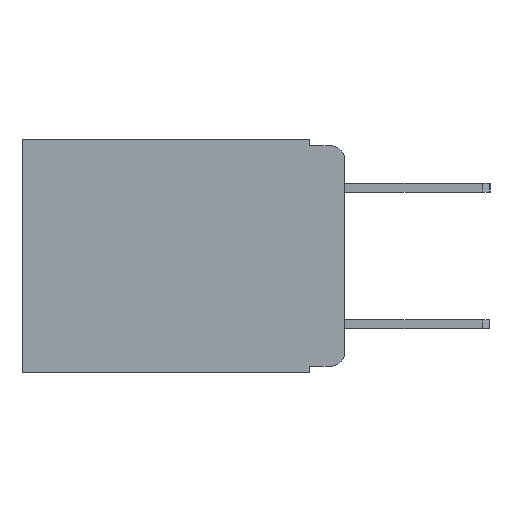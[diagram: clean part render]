
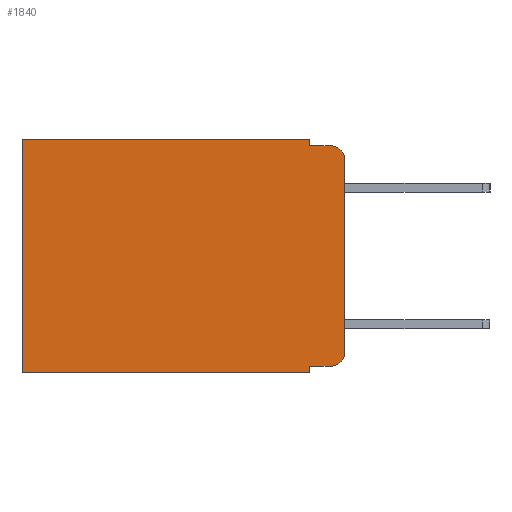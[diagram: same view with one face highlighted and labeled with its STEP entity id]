
A CAD part, left-side view. The second image highlights one B-rep face of the part: STEP entity #1840.
In plain terms, the highlighted planar face has unit normal (-1, 0, 0).
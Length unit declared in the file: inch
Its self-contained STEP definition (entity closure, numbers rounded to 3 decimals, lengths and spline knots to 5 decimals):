
#321 = ORIENTED_EDGE ( 'NONE', *, *, #17879, .T. ) ;
#538 = ORIENTED_EDGE ( 'NONE', *, *, #2535, .T. ) ;
#560 = EDGE_CURVE ( 'NONE', #4460, #9478, #13336, .T. ) ;
#1065 = DIRECTION ( 'NONE',  ( -1., 0., 0. ) ) ;
#1260 = CARTESIAN_POINT ( 'NONE',  ( 0.298, 0.051, 0. ) ) ;
#1289 = ORIENTED_EDGE ( 'NONE', *, *, #3082, .F. ) ;
#1508 = ORIENTED_EDGE ( 'NONE', *, *, #16842, .F. ) ;
#1840 = ADVANCED_FACE ( 'NONE', ( #6047 ), #12514, .F. ) ;
#1930 = ORIENTED_EDGE ( 'NONE', *, *, #10732, .T. ) ;
#2207 = DIRECTION ( 'NONE',  ( 0., 0., -1. ) ) ;
#2435 = AXIS2_PLACEMENT_3D ( 'NONE', #12482, #1065, #2207 ) ;
#2487 = VERTEX_POINT ( 'NONE', #9283 ) ;
#2535 = EDGE_CURVE ( 'NONE', #7616, #2487, #5791, .T. ) ;
#2901 = CARTESIAN_POINT ( 'NONE',  ( 0.298, 0.02, -0.333 ) ) ;
#2930 = ORIENTED_EDGE ( 'NONE', *, *, #5028, .T. ) ;
#2980 = DIRECTION ( 'NONE',  ( 0., 0., -1. ) ) ;
#3056 = EDGE_CURVE ( 'NONE', #16772, #5323, #15307, .T. ) ;
#3082 = EDGE_CURVE ( 'NONE', #16664, #2487, #7813, .T. ) ;
#3598 = CARTESIAN_POINT ( 'NONE',  ( 0.298, 0.051, -0.01 ) ) ;
#3808 = VECTOR ( 'NONE', #9976, 39.37008 ) ;
#4330 = LINE ( 'NONE', #16898, #7818 ) ;
#4460 = VERTEX_POINT ( 'NONE', #10385 ) ;
#4520 = CARTESIAN_POINT ( 'NONE',  ( 0.298, 0.051, 0. ) ) ;
#5028 = EDGE_CURVE ( 'NONE', #5469, #15815, #16810, .T. ) ;
#5250 = EDGE_LOOP ( 'NONE', ( #15176, #15580, #11083, #11491, #321, #538, #1289, #1508, #1930, #2930 ) ) ;
#5323 = VERTEX_POINT ( 'NONE', #12363 ) ;
#5452 = EDGE_CURVE ( 'NONE', #4460, #15815, #17604, .T. ) ;
#5469 = VERTEX_POINT ( 'NONE', #2901 ) ;
#5500 = VECTOR ( 'NONE', #2980, 39.37008 ) ;
#5740 = CARTESIAN_POINT ( 'NONE',  ( 0.298, 0.051, -0.343 ) ) ;
#5791 = LINE ( 'NONE', #6380, #9594 ) ;
#6042 = CARTESIAN_POINT ( 'NONE',  ( 0.298, 0., 0. ) ) ;
#6047 = FACE_OUTER_BOUND ( 'NONE', #5250, .T. ) ;
#6196 = EDGE_CURVE ( 'NONE', #5323, #9478, #10056, .T. ) ;
#6380 = CARTESIAN_POINT ( 'NONE',  ( 0.298, 0.473, 0. ) ) ;
#6411 = DIRECTION ( 'NONE',  ( 0., 0., -1. ) ) ;
#6640 = CARTESIAN_POINT ( 'NONE',  ( 0.298, 0., -0.313 ) ) ;
#6950 = CARTESIAN_POINT ( 'NONE',  ( 0.298, 0.051, 0. ) ) ;
#7023 = VECTOR ( 'NONE', #14177, 39.37008 ) ;
#7038 = DIRECTION ( 'NONE',  ( 0., 0., -1. ) ) ;
#7078 = VECTOR ( 'NONE', #9810, 39.37008 ) ;
#7616 = VERTEX_POINT ( 'NONE', #15368 ) ;
#7813 = LINE ( 'NONE', #14755, #3808 ) ;
#7818 = VECTOR ( 'NONE', #9133, 39.37008 ) ;
#8032 = AXIS2_PLACEMENT_3D ( 'NONE', #16397, #12651, #12625 ) ;
#8724 = VECTOR ( 'NONE', #7038, 39.37008 ) ;
#9133 = DIRECTION ( 'NONE',  ( 0., -1., 0. ) ) ;
#9283 = CARTESIAN_POINT ( 'NONE',  ( 0.298, 0.473, -0.343 ) ) ;
#9478 = VERTEX_POINT ( 'NONE', #14323 ) ;
#9594 = VECTOR ( 'NONE', #6411, 39.37008 ) ;
#9645 = VECTOR ( 'NONE', #12471, 39.37008 ) ;
#9765 = LINE ( 'NONE', #4520, #5500 ) ;
#9810 = DIRECTION ( 'NONE',  ( 0., 1., 0. ) ) ;
#9976 = DIRECTION ( 'NONE',  ( 0., 1., 0. ) ) ;
#10056 = LINE ( 'NONE', #3598, #9645 ) ;
#10376 = DIRECTION ( 'NONE',  ( -1., 0., 0. ) ) ;
#10385 = CARTESIAN_POINT ( 'NONE',  ( 0.298, 0., -0.03 ) ) ;
#10732 = EDGE_CURVE ( 'NONE', #13286, #5469, #4330, .T. ) ;
#11083 = ORIENTED_EDGE ( 'NONE', *, *, #6196, .F. ) ;
#11491 = ORIENTED_EDGE ( 'NONE', *, *, #3056, .F. ) ;
#12363 = CARTESIAN_POINT ( 'NONE',  ( 0.298, 0.051, -0.01 ) ) ;
#12471 = DIRECTION ( 'NONE',  ( 0., -1., 0. ) ) ;
#12482 = CARTESIAN_POINT ( 'NONE',  ( 0.298, 0.02, -0.03 ) ) ;
#12514 = PLANE ( 'NONE',  #8032 ) ;
#12625 = DIRECTION ( 'NONE',  ( 0., 0., -1. ) ) ;
#12651 = DIRECTION ( 'NONE',  ( 1., 0., 0. ) ) ;
#13286 = VERTEX_POINT ( 'NONE', #15533 ) ;
#13336 = CIRCLE ( 'NONE', #2435, 0.02 ) ;
#14177 = DIRECTION ( 'NONE',  ( 0., 0., -1. ) ) ;
#14323 = CARTESIAN_POINT ( 'NONE',  ( 0.298, 0.02, -0.01 ) ) ;
#14755 = CARTESIAN_POINT ( 'NONE',  ( 0.298, 0., -0.343 ) ) ;
#15176 = ORIENTED_EDGE ( 'NONE', *, *, #5452, .F. ) ;
#15307 = LINE ( 'NONE', #6950, #8724 ) ;
#15368 = CARTESIAN_POINT ( 'NONE',  ( 0.298, 0.473, 0. ) ) ;
#15533 = CARTESIAN_POINT ( 'NONE',  ( 0.298, 0.051, -0.333 ) ) ;
#15580 = ORIENTED_EDGE ( 'NONE', *, *, #560, .T. ) ;
#15587 = DIRECTION ( 'NONE',  ( 0., 0., -1. ) ) ;
#15815 = VERTEX_POINT ( 'NONE', #6640 ) ;
#16397 = CARTESIAN_POINT ( 'NONE',  ( 0.298, 0., 0. ) ) ;
#16664 = VERTEX_POINT ( 'NONE', #5740 ) ;
#16772 = VERTEX_POINT ( 'NONE', #1260 ) ;
#16788 = AXIS2_PLACEMENT_3D ( 'NONE', #18171, #10376, #15587 ) ;
#16810 = CIRCLE ( 'NONE', #16788, 0.02 ) ;
#16842 = EDGE_CURVE ( 'NONE', #13286, #16664, #9765, .T. ) ;
#16898 = CARTESIAN_POINT ( 'NONE',  ( 0.298, 0.051, -0.333 ) ) ;
#17598 = CARTESIAN_POINT ( 'NONE',  ( 0.298, 0., 0. ) ) ;
#17604 = LINE ( 'NONE', #6042, #7023 ) ;
#17651 = LINE ( 'NONE', #17598, #7078 ) ;
#17879 = EDGE_CURVE ( 'NONE', #16772, #7616, #17651, .T. ) ;
#18171 = CARTESIAN_POINT ( 'NONE',  ( 0.298, 0.02, -0.313 ) ) ;
